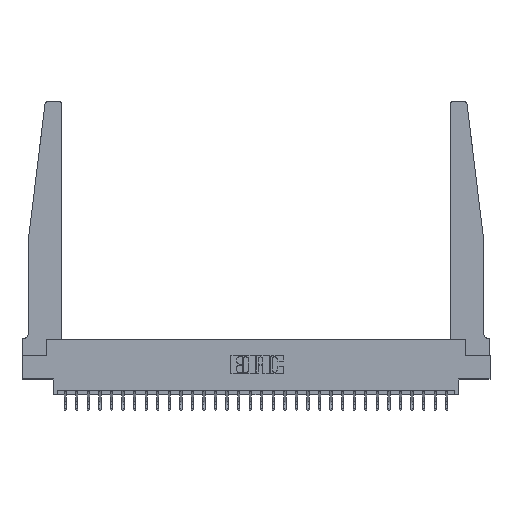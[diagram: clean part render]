
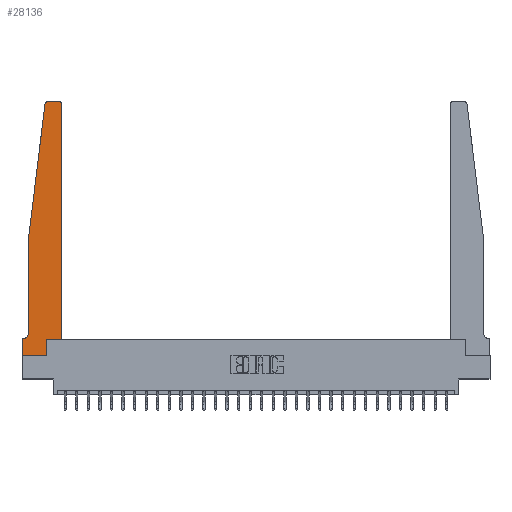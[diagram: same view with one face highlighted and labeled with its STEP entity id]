
A CAD part, top view. The second image highlights one B-rep face of the part: STEP entity #28136.
In plain terms, the highlighted planar face has unit normal (0, 0, 1).
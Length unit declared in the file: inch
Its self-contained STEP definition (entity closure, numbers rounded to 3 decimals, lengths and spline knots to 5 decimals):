
#175 = VERTEX_POINT ( 'NONE', #11834 ) ;
#237 = LINE ( 'NONE', #9109, #14267 ) ;
#657 = AXIS2_PLACEMENT_3D ( 'NONE', #4154, #19478, #1665 ) ;
#1071 = LINE ( 'NONE', #27365, #13983 ) ;
#1372 = VERTEX_POINT ( 'NONE', #26439 ) ;
#1377 = EDGE_LOOP ( 'NONE', ( #15337, #18641, #4117, #17878, #4171, #1501, #6974, #16843, #22085, #20901, #4145, #27221 ) ) ;
#1501 = ORIENTED_EDGE ( 'NONE', *, *, #7858, .T. ) ;
#1532 = AXIS2_PLACEMENT_3D ( 'NONE', #15652, #24126, #17555 ) ;
#1665 = DIRECTION ( 'NONE',  ( 1., 0., 0. ) ) ;
#1859 = VECTOR ( 'NONE', #17657, 39.37008 ) ;
#2362 = LINE ( 'NONE', #13143, #22684 ) ;
#2714 = CARTESIAN_POINT ( 'NONE',  ( 0.2605, 0.18, 0.37 ) ) ;
#2995 = EDGE_CURVE ( 'NONE', #1372, #21794, #2362, .T. ) ;
#3020 = CARTESIAN_POINT ( 'NONE',  ( 0.425, 0.18, 0.37 ) ) ;
#3078 = DIRECTION ( 'NONE',  ( 0., 0., 1. ) ) ;
#3373 = CARTESIAN_POINT ( 'NONE',  ( 0., 0.1875, 0.37 ) ) ;
#4117 = ORIENTED_EDGE ( 'NONE', *, *, #6716, .T. ) ;
#4145 = ORIENTED_EDGE ( 'NONE', *, *, #2995, .T. ) ;
#4154 = CARTESIAN_POINT ( 'NONE',  ( 0.27653, 2.72, 0.37 ) ) ;
#4171 = ORIENTED_EDGE ( 'NONE', *, *, #26368, .T. ) ;
#4661 = LINE ( 'NONE', #3020, #7162 ) ;
#6023 = CARTESIAN_POINT ( 'NONE',  ( 0., 0., 0.37 ) ) ;
#6397 = CARTESIAN_POINT ( 'NONE',  ( 0., 0.1875, 0.37 ) ) ;
#6716 = EDGE_CURVE ( 'NONE', #24014, #175, #1071, .T. ) ;
#6974 = ORIENTED_EDGE ( 'NONE', *, *, #16243, .T. ) ;
#7162 = VECTOR ( 'NONE', #9164, 39.37008 ) ;
#7583 = CARTESIAN_POINT ( 'NONE',  ( 0.425, 2.72, 0.37 ) ) ;
#7786 = DIRECTION ( 'NONE',  ( -0.122, -0.992, 0. ) ) ;
#7858 = EDGE_CURVE ( 'NONE', #20621, #11154, #237, .T. ) ;
#8478 = CARTESIAN_POINT ( 'NONE',  ( 0., 0., 0.37 ) ) ;
#8587 = VECTOR ( 'NONE', #9244, 39.37008 ) ;
#9109 = CARTESIAN_POINT ( 'NONE',  ( 0.065, 0.1875, 0.37 ) ) ;
#9164 = DIRECTION ( 'NONE',  ( 1., 0., 0. ) ) ;
#9244 = DIRECTION ( 'NONE',  ( 0., -1., 0. ) ) ;
#9541 = VERTEX_POINT ( 'NONE', #11695 ) ;
#11154 = VERTEX_POINT ( 'NONE', #6397 ) ;
#11552 = DIRECTION ( 'NONE',  ( 0., 1., 0. ) ) ;
#11695 = CARTESIAN_POINT ( 'NONE',  ( 0.2605, 0., 0.37 ) ) ;
#11834 = CARTESIAN_POINT ( 'NONE',  ( 0.065, 1.25, 0.37 ) ) ;
#11960 = VECTOR ( 'NONE', #12869, 39.37008 ) ;
#11984 = DIRECTION ( 'NONE',  ( 1., 0., 0. ) ) ;
#12005 = VECTOR ( 'NONE', #24985, 39.37008 ) ;
#12423 = VERTEX_POINT ( 'NONE', #15185 ) ;
#12610 = DIRECTION ( 'NONE',  ( -1., 0., 0. ) ) ;
#12676 = CIRCLE ( 'NONE', #18749, 0.05 ) ;
#12869 = DIRECTION ( 'NONE',  ( 1., 0., 0. ) ) ;
#12952 = VERTEX_POINT ( 'NONE', #2714 ) ;
#13143 = CARTESIAN_POINT ( 'NONE',  ( 0.425, 0.18, 0.37 ) ) ;
#13218 = CIRCLE ( 'NONE', #657, 0.03 ) ;
#13671 = VERTEX_POINT ( 'NONE', #8478 ) ;
#13983 = VECTOR ( 'NONE', #7786, 39.37008 ) ;
#14109 = CIRCLE ( 'NONE', #1532, 0.03 ) ;
#14267 = VECTOR ( 'NONE', #18033, 39.37008 ) ;
#14390 = CARTESIAN_POINT ( 'NONE',  ( 0.395, 2.75, 0.37 ) ) ;
#14528 = DIRECTION ( 'NONE',  ( -1., 0., 0. ) ) ;
#15185 = CARTESIAN_POINT ( 'NONE',  ( 0.27653, 2.75, 0.37 ) ) ;
#15195 = CARTESIAN_POINT ( 'NONE',  ( 0.24675, 2.72367, 0.37 ) ) ;
#15248 = VECTOR ( 'NONE', #12610, 39.37008 ) ;
#15337 = ORIENTED_EDGE ( 'NONE', *, *, #19833, .T. ) ;
#15344 = EDGE_CURVE ( 'NONE', #12952, #1372, #4661, .T. ) ;
#15507 = LINE ( 'NONE', #23054, #8587 ) ;
#15652 = CARTESIAN_POINT ( 'NONE',  ( 0.395, 2.72, 0.37 ) ) ;
#16160 = EDGE_CURVE ( 'NONE', #12423, #24014, #13218, .T. ) ;
#16243 = EDGE_CURVE ( 'NONE', #11154, #13671, #15507, .T. ) ;
#16843 = ORIENTED_EDGE ( 'NONE', *, *, #19027, .T. ) ;
#16968 = AXIS2_PLACEMENT_3D ( 'NONE', #3373, #3078, #11984 ) ;
#17118 = LINE ( 'NONE', #6023, #11960 ) ;
#17476 = CARTESIAN_POINT ( 'NONE',  ( 0.065, 0.2375, 0.37 ) ) ;
#17555 = DIRECTION ( 'NONE',  ( 1., 0., 0. ) ) ;
#17657 = DIRECTION ( 'NONE',  ( 0., 1., 0. ) ) ;
#17878 = ORIENTED_EDGE ( 'NONE', *, *, #21638, .T. ) ;
#18033 = DIRECTION ( 'NONE',  ( -1., 0., 0. ) ) ;
#18641 = ORIENTED_EDGE ( 'NONE', *, *, #16160, .T. ) ;
#18749 = AXIS2_PLACEMENT_3D ( 'NONE', #25639, #27264, #14528 ) ;
#19027 = EDGE_CURVE ( 'NONE', #13671, #9541, #17118, .T. ) ;
#19478 = DIRECTION ( 'NONE',  ( 0., 0., 1. ) ) ;
#19681 = CARTESIAN_POINT ( 'NONE',  ( 0.015, 0.1875, 0.37 ) ) ;
#19833 = EDGE_CURVE ( 'NONE', #25042, #12423, #28239, .T. ) ;
#20290 = LINE ( 'NONE', #26569, #1859 ) ;
#20621 = VERTEX_POINT ( 'NONE', #19681 ) ;
#20901 = ORIENTED_EDGE ( 'NONE', *, *, #15344, .T. ) ;
#21638 = EDGE_CURVE ( 'NONE', #175, #24744, #28535, .T. ) ;
#21794 = VERTEX_POINT ( 'NONE', #7583 ) ;
#22085 = ORIENTED_EDGE ( 'NONE', *, *, #24455, .T. ) ;
#22684 = VECTOR ( 'NONE', #11552, 39.37008 ) ;
#22773 = CARTESIAN_POINT ( 'NONE',  ( 0.065, 1.25, 0.37 ) ) ;
#23054 = CARTESIAN_POINT ( 'NONE',  ( 0., 0., 0.37 ) ) ;
#24014 = VERTEX_POINT ( 'NONE', #15195 ) ;
#24126 = DIRECTION ( 'NONE',  ( 0., 0., 1. ) ) ;
#24141 = CARTESIAN_POINT ( 'NONE',  ( 0.25, 2.75, 0.37 ) ) ;
#24455 = EDGE_CURVE ( 'NONE', #9541, #12952, #20290, .T. ) ;
#24744 = VERTEX_POINT ( 'NONE', #17476 ) ;
#24985 = DIRECTION ( 'NONE',  ( 0., -1., 0. ) ) ;
#25042 = VERTEX_POINT ( 'NONE', #14390 ) ;
#25639 = CARTESIAN_POINT ( 'NONE',  ( 0.015, 0.2375, 0.37 ) ) ;
#26368 = EDGE_CURVE ( 'NONE', #24744, #20621, #12676, .T. ) ;
#26439 = CARTESIAN_POINT ( 'NONE',  ( 0.425, 0.18, 0.37 ) ) ;
#26569 = CARTESIAN_POINT ( 'NONE',  ( 0.2605, 0.18, 0.37 ) ) ;
#26965 = EDGE_CURVE ( 'NONE', #21794, #25042, #14109, .T. ) ;
#27221 = ORIENTED_EDGE ( 'NONE', *, *, #26965, .T. ) ;
#27264 = DIRECTION ( 'NONE',  ( 0., 0., -1. ) ) ;
#27365 = CARTESIAN_POINT ( 'NONE',  ( 0.065, 1.25, 0.37 ) ) ;
#27476 = PLANE ( 'NONE',  #16968 ) ;
#27764 = FACE_OUTER_BOUND ( 'NONE', #1377, .T. ) ;
#28136 = ADVANCED_FACE ( 'NONE', ( #27764 ), #27476, .T. ) ;
#28239 = LINE ( 'NONE', #24141, #15248 ) ;
#28535 = LINE ( 'NONE', #22773, #12005 ) ;
